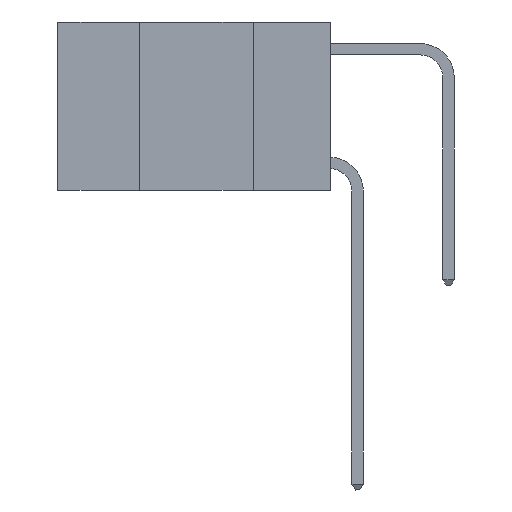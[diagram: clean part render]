
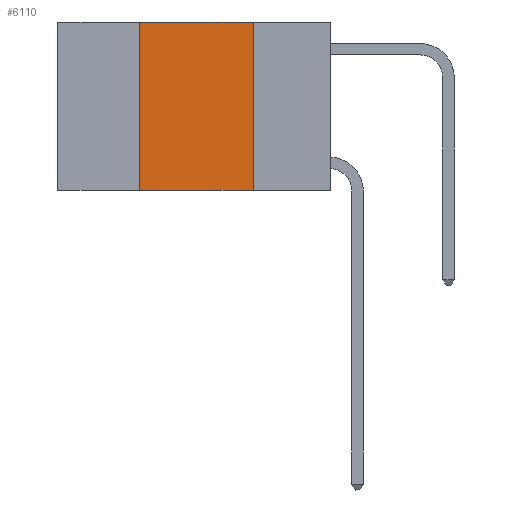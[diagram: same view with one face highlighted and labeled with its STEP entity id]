
A CAD part, left-side view. The second image highlights one B-rep face of the part: STEP entity #6110.
In plain terms, the highlighted planar face has unit normal (-1, 0, 0).
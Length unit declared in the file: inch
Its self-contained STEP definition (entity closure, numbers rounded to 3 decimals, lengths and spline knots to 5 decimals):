
#378 = CARTESIAN_POINT ( 'NONE',  ( 0., 0.6, 0. ) ) ;
#412 = VECTOR ( 'NONE', #3152, 39.37008 ) ;
#463 = CARTESIAN_POINT ( 'NONE',  ( 0., 0.17, 0. ) ) ;
#564 = EDGE_LOOP ( 'NONE', ( #6007, #9454, #10619, #7436 ) ) ;
#626 = CARTESIAN_POINT ( 'NONE',  ( 0., 0.42, 0. ) ) ;
#1060 = CARTESIAN_POINT ( 'NONE',  ( 0., 0.42, 0. ) ) ;
#2039 = DIRECTION ( 'NONE',  ( 0., 0., -1. ) ) ;
#2138 = DIRECTION ( 'NONE',  ( 0., -1., 0. ) ) ;
#2297 = CARTESIAN_POINT ( 'NONE',  ( 0., 0.17, -0.37 ) ) ;
#2738 = CARTESIAN_POINT ( 'NONE',  ( 0., 0.17, 0. ) ) ;
#2787 = PLANE ( 'NONE',  #4518 ) ;
#2793 = CARTESIAN_POINT ( 'NONE',  ( 0., 0.42, -0.37 ) ) ;
#2938 = LINE ( 'NONE', #378, #10445 ) ;
#3152 = DIRECTION ( 'NONE',  ( 0., -1., 0. ) ) ;
#3274 = CARTESIAN_POINT ( 'NONE',  ( 0., 0.6, -0.37 ) ) ;
#3362 = EDGE_CURVE ( 'NONE', #6998, #8014, #6830, .T. ) ;
#3838 = DIRECTION ( 'NONE',  ( 0., 0., 1. ) ) ;
#4395 = DIRECTION ( 'NONE',  ( 0., 0., -1. ) ) ;
#4518 = AXIS2_PLACEMENT_3D ( 'NONE', #9551, #9606, #2039 ) ;
#5287 = EDGE_CURVE ( 'NONE', #8970, #5554, #6314, .T. ) ;
#5554 = VERTEX_POINT ( 'NONE', #1060 ) ;
#5582 = LINE ( 'NONE', #3274, #412 ) ;
#6007 = ORIENTED_EDGE ( 'NONE', *, *, #3362, .F. ) ;
#6110 = ADVANCED_FACE ( 'NONE', ( #6292 ), #2787, .F. ) ;
#6292 = FACE_OUTER_BOUND ( 'NONE', #564, .T. ) ;
#6314 = LINE ( 'NONE', #626, #8988 ) ;
#6830 = LINE ( 'NONE', #2738, #7059 ) ;
#6998 = VERTEX_POINT ( 'NONE', #463 ) ;
#7059 = VECTOR ( 'NONE', #4395, 39.37008 ) ;
#7436 = ORIENTED_EDGE ( 'NONE', *, *, #8015, .T. ) ;
#7735 = EDGE_CURVE ( 'NONE', #5554, #6998, #2938, .T. ) ;
#8014 = VERTEX_POINT ( 'NONE', #2297 ) ;
#8015 = EDGE_CURVE ( 'NONE', #8970, #8014, #5582, .T. ) ;
#8970 = VERTEX_POINT ( 'NONE', #2793 ) ;
#8988 = VECTOR ( 'NONE', #3838, 39.37008 ) ;
#9454 = ORIENTED_EDGE ( 'NONE', *, *, #7735, .F. ) ;
#9551 = CARTESIAN_POINT ( 'NONE',  ( 0., 0.6, 0. ) ) ;
#9606 = DIRECTION ( 'NONE',  ( 1., 0., 0. ) ) ;
#10445 = VECTOR ( 'NONE', #2138, 39.37008 ) ;
#10619 = ORIENTED_EDGE ( 'NONE', *, *, #5287, .F. ) ;
